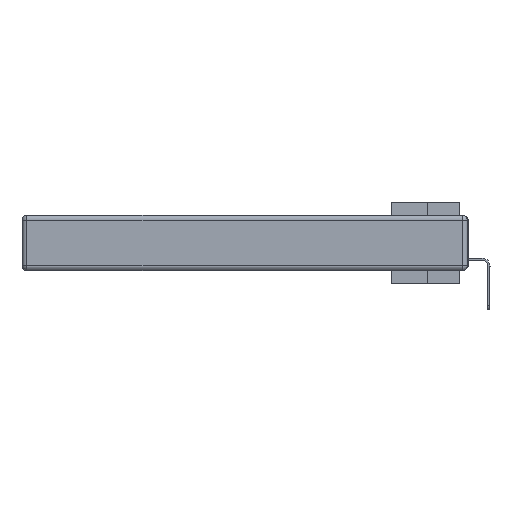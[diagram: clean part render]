
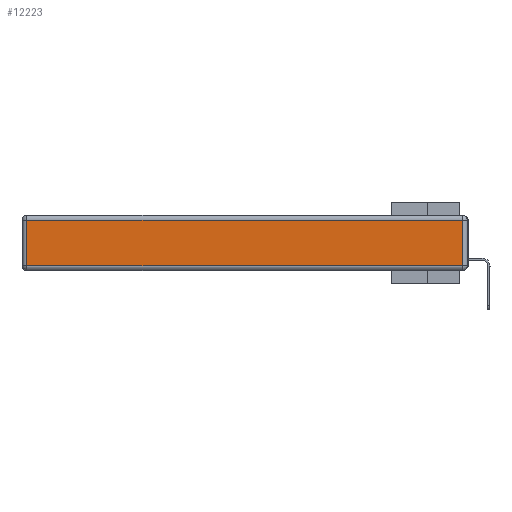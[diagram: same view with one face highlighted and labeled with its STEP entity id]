
A CAD part, left-side view. The second image highlights one B-rep face of the part: STEP entity #12223.
In plain terms, the highlighted planar face has unit normal (-1, 0, 0).
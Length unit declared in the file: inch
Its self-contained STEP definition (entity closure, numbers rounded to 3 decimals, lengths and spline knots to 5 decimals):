
#46 = VERTEX_POINT ( 'NONE', #26889 ) ;
#294 = DIRECTION ( 'NONE',  ( 0., 0., -1. ) ) ;
#840 = VECTOR ( 'NONE', #20929, 39.37008 ) ;
#854 = CARTESIAN_POINT ( 'NONE',  ( 0., 0., -0.313 ) ) ;
#1221 = EDGE_LOOP ( 'NONE', ( #10833, #18485, #35461, #28517 ) ) ;
#2342 = EDGE_CURVE ( 'NONE', #29705, #46, #14558, .T. ) ;
#3524 = CARTESIAN_POINT ( 'NONE',  ( 0., 2.72, -0.313 ) ) ;
#5798 = PLANE ( 'NONE',  #13352 ) ;
#6120 = VERTEX_POINT ( 'NONE', #3524 ) ;
#6407 = LINE ( 'NONE', #21250, #26744 ) ;
#6894 = VECTOR ( 'NONE', #33353, 39.37008 ) ;
#8499 = LINE ( 'NONE', #854, #840 ) ;
#8866 = EDGE_CURVE ( 'NONE', #31544, #6120, #13788, .T. ) ;
#9094 = CARTESIAN_POINT ( 'NONE',  ( 0., 2.72, -0.343 ) ) ;
#9465 = CARTESIAN_POINT ( 'NONE',  ( 0., 0.03, -0.343 ) ) ;
#10833 = ORIENTED_EDGE ( 'NONE', *, *, #12206, .T. ) ;
#12206 = EDGE_CURVE ( 'NONE', #6120, #29705, #8499, .T. ) ;
#12223 = ADVANCED_FACE ( 'NONE', ( #37423 ), #5798, .T. ) ;
#12321 = CARTESIAN_POINT ( 'NONE',  ( 0., 0., -0.343 ) ) ;
#13352 = AXIS2_PLACEMENT_3D ( 'NONE', #12321, #32802, #23981 ) ;
#13788 = LINE ( 'NONE', #9094, #28287 ) ;
#14558 = LINE ( 'NONE', #9465, #6894 ) ;
#16286 = DIRECTION ( 'NONE',  ( 0., 1., 0. ) ) ;
#18485 = ORIENTED_EDGE ( 'NONE', *, *, #2342, .T. ) ;
#20929 = DIRECTION ( 'NONE',  ( 0., -1., 0. ) ) ;
#21250 = CARTESIAN_POINT ( 'NONE',  ( 0., 2.75, -0.03 ) ) ;
#21260 = CARTESIAN_POINT ( 'NONE',  ( 0., 2.72, -0.03 ) ) ;
#23981 = DIRECTION ( 'NONE',  ( 0., 0., 1. ) ) ;
#26744 = VECTOR ( 'NONE', #16286, 39.37008 ) ;
#26889 = CARTESIAN_POINT ( 'NONE',  ( 0., 0.03, -0.03 ) ) ;
#28287 = VECTOR ( 'NONE', #294, 39.37008 ) ;
#28517 = ORIENTED_EDGE ( 'NONE', *, *, #8866, .T. ) ;
#29705 = VERTEX_POINT ( 'NONE', #37221 ) ;
#31544 = VERTEX_POINT ( 'NONE', #21260 ) ;
#32802 = DIRECTION ( 'NONE',  ( -1., 0., 0. ) ) ;
#33353 = DIRECTION ( 'NONE',  ( 0., 0., 1. ) ) ;
#35461 = ORIENTED_EDGE ( 'NONE', *, *, #36414, .T. ) ;
#36414 = EDGE_CURVE ( 'NONE', #46, #31544, #6407, .T. ) ;
#37221 = CARTESIAN_POINT ( 'NONE',  ( 0., 0.03, -0.313 ) ) ;
#37423 = FACE_OUTER_BOUND ( 'NONE', #1221, .T. ) ;
